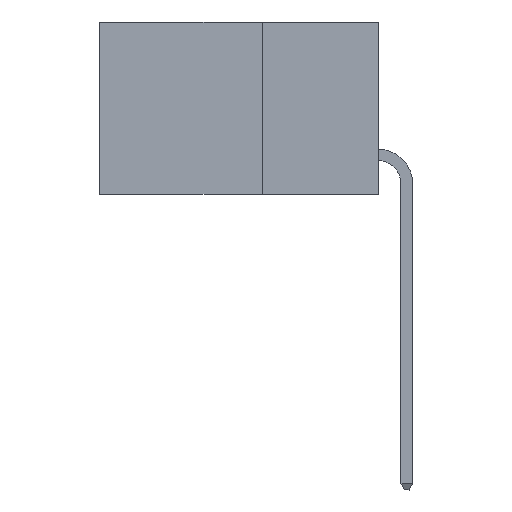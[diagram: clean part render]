
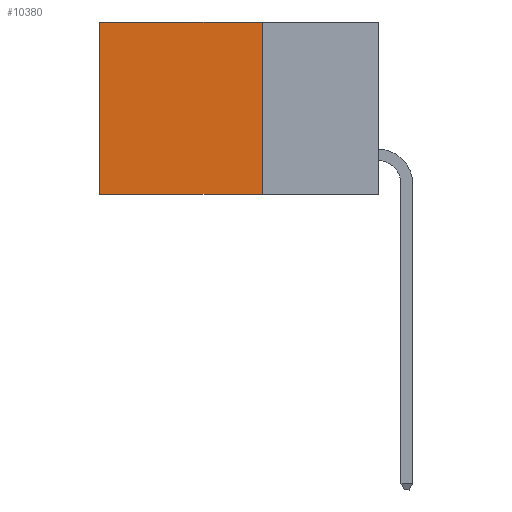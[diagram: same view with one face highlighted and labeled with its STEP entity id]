
A CAD part, left-side view. The second image highlights one B-rep face of the part: STEP entity #10380.
In plain terms, the highlighted planar face has unit normal (-1, 0, 0).
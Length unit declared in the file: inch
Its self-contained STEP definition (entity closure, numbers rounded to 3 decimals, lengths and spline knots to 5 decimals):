
#54 = CARTESIAN_POINT ( 'NONE',  ( 0.2615, 0.25, -0.37 ) ) ;
#846 = VECTOR ( 'NONE', #4599, 39.37008 ) ;
#1187 = EDGE_CURVE ( 'NONE', #7720, #5026, #7615, .T. ) ;
#1206 = LINE ( 'NONE', #1516, #5021 ) ;
#1273 = EDGE_LOOP ( 'NONE', ( #8409, #6882, #3213, #10231 ) ) ;
#1516 = CARTESIAN_POINT ( 'NONE',  ( 0.2615, 0.25, 0. ) ) ;
#2130 = DIRECTION ( 'NONE',  ( 0., 0., -1. ) ) ;
#3030 = VECTOR ( 'NONE', #2130, 39.37008 ) ;
#3213 = ORIENTED_EDGE ( 'NONE', *, *, #1187, .F. ) ;
#3378 = LINE ( 'NONE', #7758, #846 ) ;
#3628 = VERTEX_POINT ( 'NONE', #11219 ) ;
#4440 = LINE ( 'NONE', #11897, #12726 ) ;
#4599 = DIRECTION ( 'NONE',  ( 0., 1., 0. ) ) ;
#5021 = VECTOR ( 'NONE', #13051, 39.37008 ) ;
#5026 = VERTEX_POINT ( 'NONE', #7212 ) ;
#5166 = EDGE_CURVE ( 'NONE', #5026, #8630, #3378, .T. ) ;
#6449 = DIRECTION ( 'NONE',  ( 1., 0., 0. ) ) ;
#6507 = DIRECTION ( 'NONE',  ( 0., 0., -1. ) ) ;
#6882 = ORIENTED_EDGE ( 'NONE', *, *, #5166, .F. ) ;
#7212 = CARTESIAN_POINT ( 'NONE',  ( 0.2615, 0.25, -0.37 ) ) ;
#7572 = CARTESIAN_POINT ( 'NONE',  ( 0.2615, 0.25, 0. ) ) ;
#7615 = LINE ( 'NONE', #54, #3030 ) ;
#7720 = VERTEX_POINT ( 'NONE', #7572 ) ;
#7758 = CARTESIAN_POINT ( 'NONE',  ( 0.2615, 0.25, -0.37 ) ) ;
#8247 = EDGE_CURVE ( 'NONE', #7720, #3628, #1206, .T. ) ;
#8305 = AXIS2_PLACEMENT_3D ( 'NONE', #10738, #6449, #6507 ) ;
#8409 = ORIENTED_EDGE ( 'NONE', *, *, #13453, .T. ) ;
#8630 = VERTEX_POINT ( 'NONE', #9301 ) ;
#9301 = CARTESIAN_POINT ( 'NONE',  ( 0.2615, 0.6, -0.37 ) ) ;
#10231 = ORIENTED_EDGE ( 'NONE', *, *, #8247, .T. ) ;
#10380 = ADVANCED_FACE ( 'NONE', ( #12514 ), #10665, .F. ) ;
#10665 = PLANE ( 'NONE',  #8305 ) ;
#10738 = CARTESIAN_POINT ( 'NONE',  ( 0.2615, 0.25, -0.37 ) ) ;
#11078 = DIRECTION ( 'NONE',  ( 0., 0., -1. ) ) ;
#11219 = CARTESIAN_POINT ( 'NONE',  ( 0.2615, 0.6, 0. ) ) ;
#11897 = CARTESIAN_POINT ( 'NONE',  ( 0.2615, 0.6, -0.37 ) ) ;
#12514 = FACE_OUTER_BOUND ( 'NONE', #1273, .T. ) ;
#12726 = VECTOR ( 'NONE', #11078, 39.37008 ) ;
#13051 = DIRECTION ( 'NONE',  ( 0., 1., 0. ) ) ;
#13453 = EDGE_CURVE ( 'NONE', #3628, #8630, #4440, .T. ) ;
